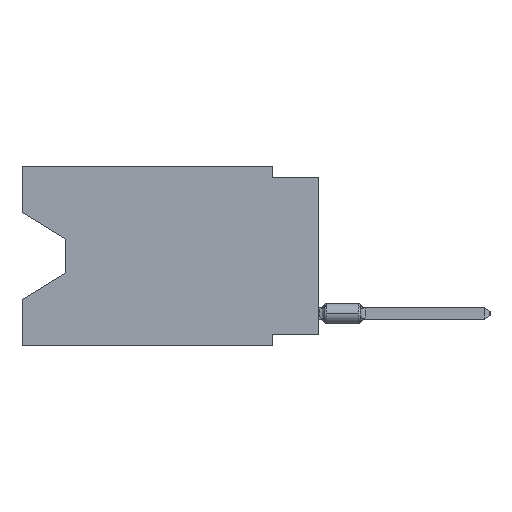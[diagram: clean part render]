
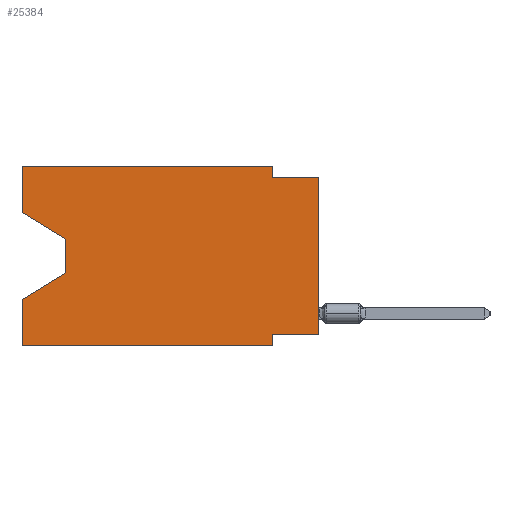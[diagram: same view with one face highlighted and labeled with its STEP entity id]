
A CAD part, left-side view. The second image highlights one B-rep face of the part: STEP entity #25384.
In plain terms, the highlighted planar face has unit normal (-1, 0, 0).
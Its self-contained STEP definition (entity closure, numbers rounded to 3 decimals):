
#153 = EDGE_CURVE ( 'NONE', #4715, #31158, #30273, .T. ) ;
#320 = CARTESIAN_POINT ( 'NONE',  ( 0., 2.54, 0. ) ) ;
#342 = DIRECTION ( 'NONE',  ( 0., -1., 0. ) ) ;
#503 = CARTESIAN_POINT ( 'NONE',  ( 0., 2.54, 0. ) ) ;
#673 = CARTESIAN_POINT ( 'NONE',  ( 0., 2.54, -9.906 ) ) ;
#694 = DIRECTION ( 'NONE',  ( 0., 0., -1. ) ) ;
#844 = CARTESIAN_POINT ( 'NONE',  ( 0., 13.97, -4.013 ) ) ;
#1230 = CARTESIAN_POINT ( 'NONE',  ( 0., 13.97, -5.893 ) ) ;
#1642 = ORIENTED_EDGE ( 'NONE', *, *, #31806, .F. ) ;
#2096 = CARTESIAN_POINT ( 'NONE',  ( 0., 0., -9.271 ) ) ;
#2398 = ORIENTED_EDGE ( 'NONE', *, *, #24004, .T. ) ;
#2656 = ORIENTED_EDGE ( 'NONE', *, *, #17110, .F. ) ;
#3195 = DIRECTION ( 'NONE',  ( 0., -1., 0. ) ) ;
#3381 = CARTESIAN_POINT ( 'NONE',  ( 0., 0., -0.635 ) ) ;
#3765 = FACE_OUTER_BOUND ( 'NONE', #37022, .T. ) ;
#4154 = VECTOR ( 'NONE', #342, 1000. ) ;
#4199 = DIRECTION ( 'NONE',  ( 0., 0., -1. ) ) ;
#4402 = CARTESIAN_POINT ( 'NONE',  ( 0., 16.383, -7.36 ) ) ;
#4683 = LINE ( 'NONE', #17282, #27196 ) ;
#4715 = VERTEX_POINT ( 'NONE', #35126 ) ;
#4862 = CARTESIAN_POINT ( 'NONE',  ( 0., 16.383, -2.546 ) ) ;
#5323 = LINE ( 'NONE', #14669, #9815 ) ;
#5336 = EDGE_CURVE ( 'NONE', #36561, #15584, #24636, .T. ) ;
#6142 = CARTESIAN_POINT ( 'NONE',  ( 0., 0., -0.635 ) ) ;
#6493 = EDGE_CURVE ( 'NONE', #32571, #35272, #5323, .T. ) ;
#6800 = PLANE ( 'NONE',  #35380 ) ;
#6934 = VERTEX_POINT ( 'NONE', #23969 ) ;
#7820 = EDGE_CURVE ( 'NONE', #32571, #35226, #8781, .T. ) ;
#8503 = DIRECTION ( 'NONE',  ( 0., -0.855, -0.519 ) ) ;
#8586 = VERTEX_POINT ( 'NONE', #673 ) ;
#8781 = LINE ( 'NONE', #11419, #19663 ) ;
#8902 = CARTESIAN_POINT ( 'NONE',  ( 0., 16.383, 0. ) ) ;
#9004 = LINE ( 'NONE', #27922, #36581 ) ;
#9815 = VECTOR ( 'NONE', #32557, 1000. ) ;
#11419 = CARTESIAN_POINT ( 'NONE',  ( 0., 0., -9.271 ) ) ;
#12224 = EDGE_CURVE ( 'NONE', #24385, #27785, #22240, .T. ) ;
#12694 = VECTOR ( 'NONE', #21570, 1000. ) ;
#13670 = DIRECTION ( 'NONE',  ( 1., 0., 0. ) ) ;
#14669 = CARTESIAN_POINT ( 'NONE',  ( 0., 0., 0. ) ) ;
#14699 = LINE ( 'NONE', #22680, #15516 ) ;
#15093 = DIRECTION ( 'NONE',  ( 0., 0., 1. ) ) ;
#15204 = VECTOR ( 'NONE', #37541, 1000. ) ;
#15516 = VECTOR ( 'NONE', #4199, 1000. ) ;
#15584 = VERTEX_POINT ( 'NONE', #4402 ) ;
#16454 = EDGE_CURVE ( 'NONE', #6934, #24385, #4683, .T. ) ;
#16531 = CARTESIAN_POINT ( 'NONE',  ( 0., 16.383, 0. ) ) ;
#17110 = EDGE_CURVE ( 'NONE', #35226, #8586, #14699, .T. ) ;
#17282 = CARTESIAN_POINT ( 'NONE',  ( 0., 16.383, 0. ) ) ;
#17377 = ORIENTED_EDGE ( 'NONE', *, *, #12224, .F. ) ;
#17395 = LINE ( 'NONE', #23489, #23696 ) ;
#17988 = ORIENTED_EDGE ( 'NONE', *, *, #5336, .T. ) ;
#19658 = CARTESIAN_POINT ( 'NONE',  ( 0., 2.54, -0.635 ) ) ;
#19663 = VECTOR ( 'NONE', #30340, 1000. ) ;
#20883 = LINE ( 'NONE', #8902, #25454 ) ;
#21570 = DIRECTION ( 'NONE',  ( 0., 0.855, -0.519 ) ) ;
#22240 = LINE ( 'NONE', #320, #15204 ) ;
#22680 = CARTESIAN_POINT ( 'NONE',  ( 0., 2.54, -9.906 ) ) ;
#23489 = CARTESIAN_POINT ( 'NONE',  ( 0., 13.97, -4.013 ) ) ;
#23668 = CARTESIAN_POINT ( 'NONE',  ( 0., 16.383, -9.906 ) ) ;
#23696 = VECTOR ( 'NONE', #33068, 1000. ) ;
#23969 = CARTESIAN_POINT ( 'NONE',  ( 0., 16.383, 0. ) ) ;
#24004 = EDGE_CURVE ( 'NONE', #36404, #8586, #28191, .T. ) ;
#24385 = VERTEX_POINT ( 'NONE', #503 ) ;
#24636 = LINE ( 'NONE', #27703, #12694 ) ;
#24687 = ORIENTED_EDGE ( 'NONE', *, *, #6493, .T. ) ;
#25091 = VECTOR ( 'NONE', #8503, 1000. ) ;
#25384 = ADVANCED_FACE ( 'NONE', ( #3765 ), #6800, .F. ) ;
#25454 = VECTOR ( 'NONE', #33302, 1000. ) ;
#27196 = VECTOR ( 'NONE', #39053, 1000. ) ;
#27703 = CARTESIAN_POINT ( 'NONE',  ( 0., 13.97, -5.893 ) ) ;
#27785 = VERTEX_POINT ( 'NONE', #19658 ) ;
#27922 = CARTESIAN_POINT ( 'NONE',  ( 0., 16.383, 0. ) ) ;
#28191 = LINE ( 'NONE', #37944, #4154 ) ;
#29326 = VECTOR ( 'NONE', #3195, 1000. ) ;
#30273 = LINE ( 'NONE', #4862, #25091 ) ;
#30340 = DIRECTION ( 'NONE',  ( 0., 1., 0. ) ) ;
#30836 = LINE ( 'NONE', #3381, #29326 ) ;
#31158 = VERTEX_POINT ( 'NONE', #844 ) ;
#31806 = EDGE_CURVE ( 'NONE', #36404, #15584, #20883, .T. ) ;
#32557 = DIRECTION ( 'NONE',  ( 0., 0., 1. ) ) ;
#32571 = VERTEX_POINT ( 'NONE', #2096 ) ;
#32676 = EDGE_CURVE ( 'NONE', #4715, #6934, #9004, .T. ) ;
#32780 = ORIENTED_EDGE ( 'NONE', *, *, #40144, .T. ) ;
#33068 = DIRECTION ( 'NONE',  ( 0., 0., -1. ) ) ;
#33108 = ORIENTED_EDGE ( 'NONE', *, *, #32676, .F. ) ;
#33222 = ORIENTED_EDGE ( 'NONE', *, *, #36039, .F. ) ;
#33302 = DIRECTION ( 'NONE',  ( 0., 0., 1. ) ) ;
#35126 = CARTESIAN_POINT ( 'NONE',  ( 0., 16.383, -2.546 ) ) ;
#35145 = ORIENTED_EDGE ( 'NONE', *, *, #7820, .F. ) ;
#35226 = VERTEX_POINT ( 'NONE', #40108 ) ;
#35272 = VERTEX_POINT ( 'NONE', #6142 ) ;
#35380 = AXIS2_PLACEMENT_3D ( 'NONE', #16531, #13670, #694 ) ;
#36039 = EDGE_CURVE ( 'NONE', #27785, #35272, #30836, .T. ) ;
#36404 = VERTEX_POINT ( 'NONE', #23668 ) ;
#36561 = VERTEX_POINT ( 'NONE', #1230 ) ;
#36581 = VECTOR ( 'NONE', #15093, 1000. ) ;
#37022 = EDGE_LOOP ( 'NONE', ( #38462, #32780, #17988, #1642, #2398, #2656, #35145, #24687, #33222, #17377, #39686, #33108 ) ) ;
#37541 = DIRECTION ( 'NONE',  ( 0., 0., -1. ) ) ;
#37944 = CARTESIAN_POINT ( 'NONE',  ( 0., 16.383, -9.906 ) ) ;
#38462 = ORIENTED_EDGE ( 'NONE', *, *, #153, .T. ) ;
#39053 = DIRECTION ( 'NONE',  ( 0., -1., 0. ) ) ;
#39686 = ORIENTED_EDGE ( 'NONE', *, *, #16454, .F. ) ;
#40108 = CARTESIAN_POINT ( 'NONE',  ( 0., 2.54, -9.271 ) ) ;
#40144 = EDGE_CURVE ( 'NONE', #31158, #36561, #17395, .T. ) ;
